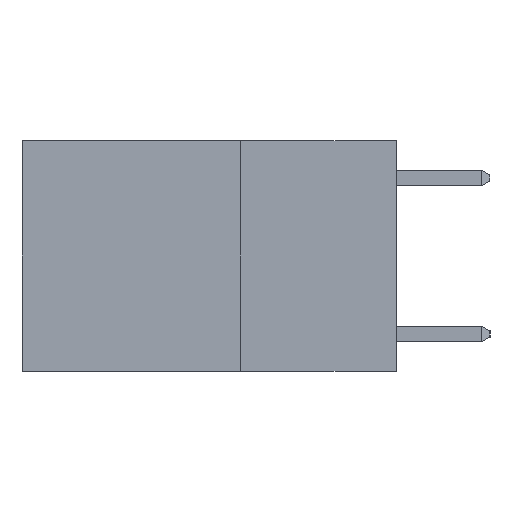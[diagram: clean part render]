
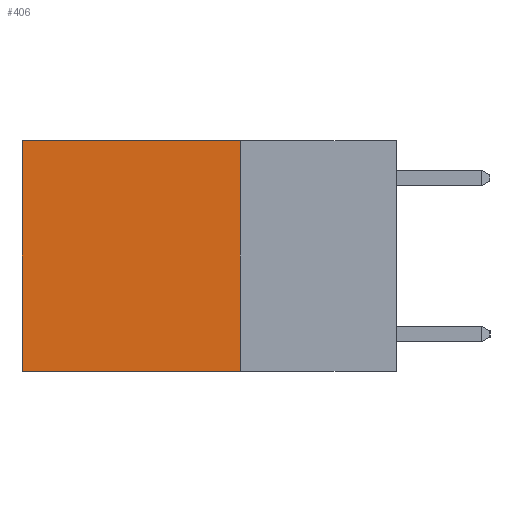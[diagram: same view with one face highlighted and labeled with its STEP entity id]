
A CAD part, left-side view. The second image highlights one B-rep face of the part: STEP entity #406.
In plain terms, the highlighted planar face has unit normal (-1, 0, 0).
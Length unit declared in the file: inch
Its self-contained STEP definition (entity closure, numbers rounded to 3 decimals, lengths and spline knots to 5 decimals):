
#406 = ADVANCED_FACE ( 'NONE', ( #7902 ), #8394, .F. ) ;
#1163 = DIRECTION ( 'NONE',  ( 0., 1., 0. ) ) ;
#1179 = CARTESIAN_POINT ( 'NONE',  ( 0.2625, 0.25, 0. ) ) ;
#1185 = DIRECTION ( 'NONE',  ( 0., 0., -1. ) ) ;
#1416 = CARTESIAN_POINT ( 'NONE',  ( 0.2625, 0.25, -0.37 ) ) ;
#1659 = ORIENTED_EDGE ( 'NONE', *, *, #3141, .F. ) ;
#1805 = DIRECTION ( 'NONE',  ( 0., 1., 0. ) ) ;
#1879 = CARTESIAN_POINT ( 'NONE',  ( 0.2625, 0.25, -0.37 ) ) ;
#2008 = LINE ( 'NONE', #1179, #6965 ) ;
#2022 = CARTESIAN_POINT ( 'NONE',  ( 0.2625, 0.6, 0. ) ) ;
#2327 = DIRECTION ( 'NONE',  ( 1., 0., 0. ) ) ;
#2380 = DIRECTION ( 'NONE',  ( 0., 0., -1. ) ) ;
#2866 = EDGE_LOOP ( 'NONE', ( #7211, #3556, #1659, #5686 ) ) ;
#3021 = VECTOR ( 'NONE', #1805, 39.37008 ) ;
#3141 = EDGE_CURVE ( 'NONE', #4527, #5356, #3634, .T. ) ;
#3556 = ORIENTED_EDGE ( 'NONE', *, *, #3709, .F. ) ;
#3610 = CARTESIAN_POINT ( 'NONE',  ( 0.2625, 0.25, 0. ) ) ;
#3634 = LINE ( 'NONE', #3610, #5323 ) ;
#3643 = DIRECTION ( 'NONE',  ( 0., 0., -1. ) ) ;
#3659 = VERTEX_POINT ( 'NONE', #2022 ) ;
#3709 = EDGE_CURVE ( 'NONE', #5356, #8360, #4712, .T. ) ;
#3875 = EDGE_CURVE ( 'NONE', #4527, #3659, #2008, .T. ) ;
#3936 = CARTESIAN_POINT ( 'NONE',  ( 0.2625, 0.6, -0.37 ) ) ;
#4253 = CARTESIAN_POINT ( 'NONE',  ( 0.2625, 0.25, 0. ) ) ;
#4527 = VERTEX_POINT ( 'NONE', #5872 ) ;
#4712 = LINE ( 'NONE', #1879, #3021 ) ;
#5304 = AXIS2_PLACEMENT_3D ( 'NONE', #4253, #2327, #1185 ) ;
#5323 = VECTOR ( 'NONE', #3643, 39.37008 ) ;
#5356 = VERTEX_POINT ( 'NONE', #1416 ) ;
#5488 = VECTOR ( 'NONE', #2380, 39.37008 ) ;
#5686 = ORIENTED_EDGE ( 'NONE', *, *, #3875, .T. ) ;
#5872 = CARTESIAN_POINT ( 'NONE',  ( 0.2625, 0.25, 0. ) ) ;
#6212 = CARTESIAN_POINT ( 'NONE',  ( 0.2625, 0.6, 0. ) ) ;
#6479 = EDGE_CURVE ( 'NONE', #3659, #8360, #6835, .T. ) ;
#6835 = LINE ( 'NONE', #6212, #5488 ) ;
#6965 = VECTOR ( 'NONE', #1163, 39.37008 ) ;
#7211 = ORIENTED_EDGE ( 'NONE', *, *, #6479, .T. ) ;
#7902 = FACE_OUTER_BOUND ( 'NONE', #2866, .T. ) ;
#8360 = VERTEX_POINT ( 'NONE', #3936 ) ;
#8394 = PLANE ( 'NONE',  #5304 ) ;
